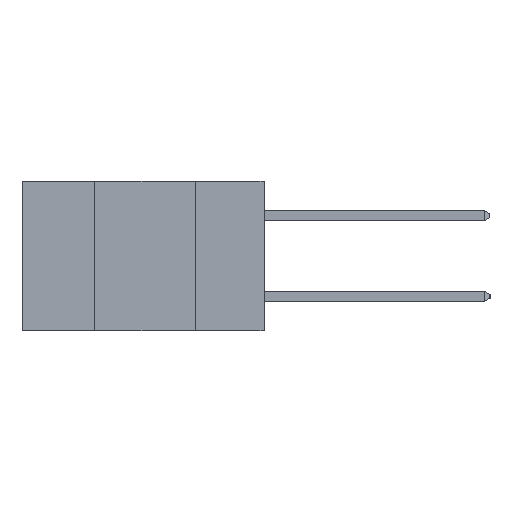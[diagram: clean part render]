
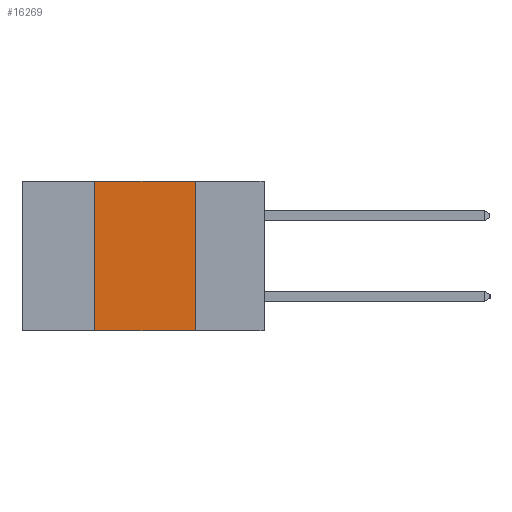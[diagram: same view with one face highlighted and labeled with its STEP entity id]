
A CAD part, left-side view. The second image highlights one B-rep face of the part: STEP entity #16269.
In plain terms, the highlighted planar face has unit normal (-1, 0, 0).
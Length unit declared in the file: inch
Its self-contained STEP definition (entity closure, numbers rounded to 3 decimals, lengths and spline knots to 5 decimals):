
#516 = EDGE_CURVE ( 'NONE', #9334, #5247, #3563, .T. ) ;
#562 = ORIENTED_EDGE ( 'NONE', *, *, #18782, .T. ) ;
#1739 = CARTESIAN_POINT ( 'NONE',  ( 0., 0.6, -0.37 ) ) ;
#1848 = ORIENTED_EDGE ( 'NONE', *, *, #3848, .F. ) ;
#2068 = CARTESIAN_POINT ( 'NONE',  ( 0., 0.17, 0. ) ) ;
#2151 = DIRECTION ( 'NONE',  ( 0., 0., -1. ) ) ;
#2504 = CARTESIAN_POINT ( 'NONE',  ( 0., 0.42, -0.37 ) ) ;
#2737 = EDGE_CURVE ( 'NONE', #5247, #11424, #3648, .T. ) ;
#2886 = ORIENTED_EDGE ( 'NONE', *, *, #2737, .F. ) ;
#3039 = VECTOR ( 'NONE', #9607, 39.37008 ) ;
#3062 = FACE_OUTER_BOUND ( 'NONE', #5876, .T. ) ;
#3563 = LINE ( 'NONE', #10428, #3039 ) ;
#3648 = LINE ( 'NONE', #8461, #16337 ) ;
#3848 = EDGE_CURVE ( 'NONE', #11424, #10774, #19789, .T. ) ;
#4897 = AXIS2_PLACEMENT_3D ( 'NONE', #5947, #19301, #9255 ) ;
#5076 = DIRECTION ( 'NONE',  ( 0., -1., 0. ) ) ;
#5247 = VERTEX_POINT ( 'NONE', #5552 ) ;
#5552 = CARTESIAN_POINT ( 'NONE',  ( 0., 0.42, 0. ) ) ;
#5876 = EDGE_LOOP ( 'NONE', ( #1848, #2886, #20109, #562 ) ) ;
#5947 = CARTESIAN_POINT ( 'NONE',  ( 0., 0.6, 0. ) ) ;
#6963 = VECTOR ( 'NONE', #2151, 39.37008 ) ;
#7592 = PLANE ( 'NONE',  #4897 ) ;
#8461 = CARTESIAN_POINT ( 'NONE',  ( 0., 0.6, 0. ) ) ;
#8860 = VECTOR ( 'NONE', #5076, 39.37008 ) ;
#9255 = DIRECTION ( 'NONE',  ( 0., 0., -1. ) ) ;
#9334 = VERTEX_POINT ( 'NONE', #2504 ) ;
#9607 = DIRECTION ( 'NONE',  ( 0., 0., 1. ) ) ;
#10428 = CARTESIAN_POINT ( 'NONE',  ( 0., 0.42, -0.37 ) ) ;
#10660 = CARTESIAN_POINT ( 'NONE',  ( 0., 0.17, -0.37 ) ) ;
#10774 = VERTEX_POINT ( 'NONE', #12133 ) ;
#11424 = VERTEX_POINT ( 'NONE', #2068 ) ;
#12133 = CARTESIAN_POINT ( 'NONE',  ( 0., 0.17, -0.37 ) ) ;
#13574 = DIRECTION ( 'NONE',  ( 0., -1., 0. ) ) ;
#16269 = ADVANCED_FACE ( 'NONE', ( #3062 ), #7592, .F. ) ;
#16337 = VECTOR ( 'NONE', #13574, 39.37008 ) ;
#17738 = LINE ( 'NONE', #1739, #8860 ) ;
#18782 = EDGE_CURVE ( 'NONE', #9334, #10774, #17738, .T. ) ;
#19301 = DIRECTION ( 'NONE',  ( 1., 0., 0. ) ) ;
#19789 = LINE ( 'NONE', #10660, #6963 ) ;
#20109 = ORIENTED_EDGE ( 'NONE', *, *, #516, .F. ) ;
